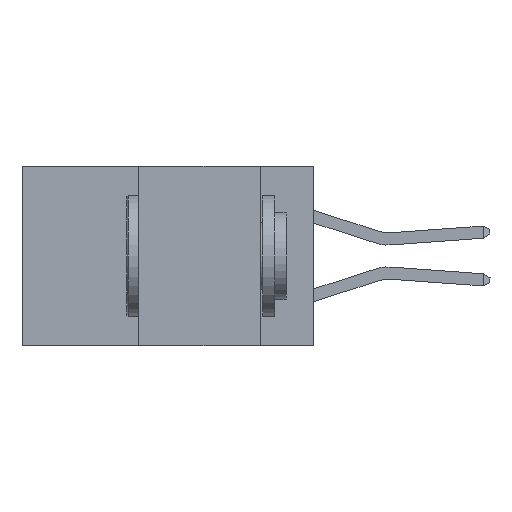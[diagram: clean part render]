
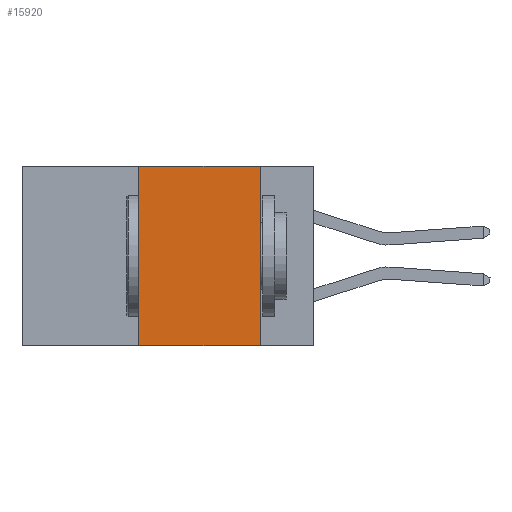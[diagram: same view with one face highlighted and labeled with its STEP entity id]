
A CAD part, left-side view. The second image highlights one B-rep face of the part: STEP entity #15920.
In plain terms, the highlighted planar face has unit normal (-1, 0, 0).
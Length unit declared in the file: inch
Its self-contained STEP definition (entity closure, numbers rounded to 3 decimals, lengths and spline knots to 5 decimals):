
#1545 = DIRECTION ( 'NONE',  ( 0., -1., 0. ) ) ;
#1769 = LINE ( 'NONE', #5676, #10601 ) ;
#2218 = DIRECTION ( 'NONE',  ( 0., -1., 0. ) ) ;
#2544 = CARTESIAN_POINT ( 'NONE',  ( 0., 0.6, 0. ) ) ;
#2990 = VERTEX_POINT ( 'NONE', #19603 ) ;
#4292 = DIRECTION ( 'NONE',  ( 1., 0., 0. ) ) ;
#5605 = ORIENTED_EDGE ( 'NONE', *, *, #15291, .F. ) ;
#5676 = CARTESIAN_POINT ( 'NONE',  ( 0., 0.6, -0.37 ) ) ;
#5822 = CARTESIAN_POINT ( 'NONE',  ( 0., 0.11, 0. ) ) ;
#5986 = AXIS2_PLACEMENT_3D ( 'NONE', #2544, #4292, #16614 ) ;
#8337 = VERTEX_POINT ( 'NONE', #17681 ) ;
#8456 = ORIENTED_EDGE ( 'NONE', *, *, #20821, .F. ) ;
#9121 = EDGE_CURVE ( 'NONE', #17583, #2990, #1769, .T. ) ;
#9877 = EDGE_CURVE ( 'NONE', #8337, #2990, #17905, .T. ) ;
#10601 = VECTOR ( 'NONE', #2218, 39.37008 ) ;
#10656 = DIRECTION ( 'NONE',  ( 0., 0., 1. ) ) ;
#10807 = CARTESIAN_POINT ( 'NONE',  ( 0., 0.36, -0.37 ) ) ;
#10891 = LINE ( 'NONE', #12112, #12006 ) ;
#11615 = CARTESIAN_POINT ( 'NONE',  ( 0., 0.36, 0. ) ) ;
#11691 = FACE_OUTER_BOUND ( 'NONE', #17163, .T. ) ;
#12006 = VECTOR ( 'NONE', #1545, 39.37008 ) ;
#12112 = CARTESIAN_POINT ( 'NONE',  ( 0., 0.6, 0. ) ) ;
#13455 = LINE ( 'NONE', #19326, #16976 ) ;
#13631 = ORIENTED_EDGE ( 'NONE', *, *, #9877, .F. ) ;
#15291 = EDGE_CURVE ( 'NONE', #19977, #8337, #10891, .T. ) ;
#15920 = ADVANCED_FACE ( 'NONE', ( #11691 ), #21733, .F. ) ;
#16614 = DIRECTION ( 'NONE',  ( 0., 0., -1. ) ) ;
#16976 = VECTOR ( 'NONE', #10656, 39.37008 ) ;
#17163 = EDGE_LOOP ( 'NONE', ( #13631, #5605, #8456, #19734 ) ) ;
#17583 = VERTEX_POINT ( 'NONE', #10807 ) ;
#17681 = CARTESIAN_POINT ( 'NONE',  ( 0., 0.11, 0. ) ) ;
#17905 = LINE ( 'NONE', #5822, #21957 ) ;
#17983 = DIRECTION ( 'NONE',  ( 0., 0., -1. ) ) ;
#19326 = CARTESIAN_POINT ( 'NONE',  ( 0., 0.36, 0. ) ) ;
#19603 = CARTESIAN_POINT ( 'NONE',  ( 0., 0.11, -0.37 ) ) ;
#19734 = ORIENTED_EDGE ( 'NONE', *, *, #9121, .T. ) ;
#19977 = VERTEX_POINT ( 'NONE', #11615 ) ;
#20821 = EDGE_CURVE ( 'NONE', #17583, #19977, #13455, .T. ) ;
#21733 = PLANE ( 'NONE',  #5986 ) ;
#21957 = VECTOR ( 'NONE', #17983, 39.37008 ) ;
